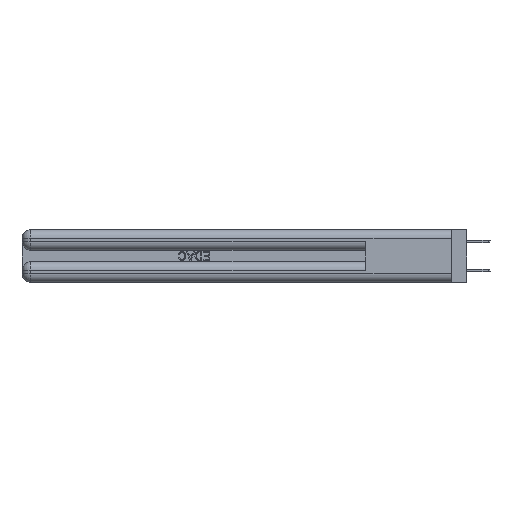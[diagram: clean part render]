
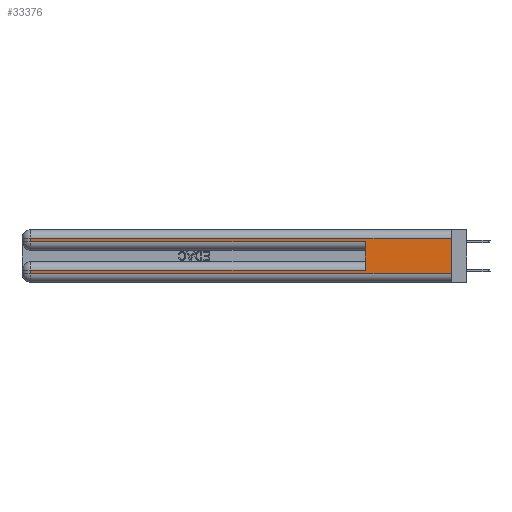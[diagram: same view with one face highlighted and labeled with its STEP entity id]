
A CAD part, left-side view. The second image highlights one B-rep face of the part: STEP entity #33376.
In plain terms, the highlighted planar face has unit normal (-1, 0, 0).
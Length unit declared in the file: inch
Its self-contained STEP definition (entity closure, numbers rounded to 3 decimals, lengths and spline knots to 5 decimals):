
#803 = LINE ( 'NONE', #3390, #34950 ) ;
#2134 = CARTESIAN_POINT ( 'NONE',  ( 0., 2.94, 0.085 ) ) ;
#2688 = VERTEX_POINT ( 'NONE', #10606 ) ;
#3357 = VECTOR ( 'NONE', #13392, 39.37008 ) ;
#3390 = CARTESIAN_POINT ( 'NONE',  ( 0., 0., 0.31 ) ) ;
#4240 = CARTESIAN_POINT ( 'NONE',  ( 0., 0., 0.37 ) ) ;
#5053 = CARTESIAN_POINT ( 'NONE',  ( 0., 2.94, 0.285 ) ) ;
#6180 = EDGE_CURVE ( 'NONE', #27935, #36361, #23320, .T. ) ;
#6785 = DIRECTION ( 'NONE',  ( 0., 1., 0. ) ) ;
#7603 = DIRECTION ( 'NONE',  ( 0., 0., -1. ) ) ;
#8574 = ORIENTED_EDGE ( 'NONE', *, *, #15622, .T. ) ;
#8674 = ORIENTED_EDGE ( 'NONE', *, *, #22740, .F. ) ;
#9617 = DIRECTION ( 'NONE',  ( 0., -1., 0. ) ) ;
#10099 = CARTESIAN_POINT ( 'NONE',  ( 0., 0.6, 0.145 ) ) ;
#10606 = CARTESIAN_POINT ( 'NONE',  ( 0., 0., 0.06 ) ) ;
#11550 = VERTEX_POINT ( 'NONE', #33632 ) ;
#13392 = DIRECTION ( 'NONE',  ( 0., 0., 1. ) ) ;
#14465 = CARTESIAN_POINT ( 'NONE',  ( 0., 2.94, 0.37 ) ) ;
#15622 = EDGE_CURVE ( 'NONE', #24489, #27935, #23528, .T. ) ;
#15987 = VERTEX_POINT ( 'NONE', #23388 ) ;
#16885 = CARTESIAN_POINT ( 'NONE',  ( 0., 0., 0.31 ) ) ;
#17407 = PLANE ( 'NONE',  #38671 ) ;
#17428 = DIRECTION ( 'NONE',  ( 0., 1., 0. ) ) ;
#18054 = EDGE_CURVE ( 'NONE', #36361, #2688, #40770, .T. ) ;
#18984 = ORIENTED_EDGE ( 'NONE', *, *, #21351, .T. ) ;
#19740 = LINE ( 'NONE', #29223, #36273 ) ;
#21266 = VECTOR ( 'NONE', #34198, 39.37008 ) ;
#21351 = EDGE_CURVE ( 'NONE', #11550, #28481, #19740, .T. ) ;
#22107 = FACE_OUTER_BOUND ( 'NONE', #23478, .T. ) ;
#22740 = EDGE_CURVE ( 'NONE', #38735, #2688, #38508, .T. ) ;
#23072 = VECTOR ( 'NONE', #37963, 39.37008 ) ;
#23320 = LINE ( 'NONE', #14465, #21266 ) ;
#23343 = CARTESIAN_POINT ( 'NONE',  ( 0., 0., 0.37 ) ) ;
#23388 = CARTESIAN_POINT ( 'NONE',  ( 0., 0.6, 0.285 ) ) ;
#23475 = DIRECTION ( 'NONE',  ( 0., 0., -1. ) ) ;
#23478 = EDGE_LOOP ( 'NONE', ( #8674, #36290, #18984, #28076, #25485, #8574, #33791, #26164 ) ) ;
#23528 = LINE ( 'NONE', #40569, #41222 ) ;
#24489 = VERTEX_POINT ( 'NONE', #25614 ) ;
#24587 = CARTESIAN_POINT ( 'NONE',  ( 0., 0., 0.06 ) ) ;
#25485 = ORIENTED_EDGE ( 'NONE', *, *, #28805, .F. ) ;
#25614 = CARTESIAN_POINT ( 'NONE',  ( 0., 0.6, 0.085 ) ) ;
#25879 = DIRECTION ( 'NONE',  ( 0., 0., -1. ) ) ;
#26164 = ORIENTED_EDGE ( 'NONE', *, *, #18054, .T. ) ;
#27282 = DIRECTION ( 'NONE',  ( 1., 0., 0. ) ) ;
#27935 = VERTEX_POINT ( 'NONE', #2134 ) ;
#28076 = ORIENTED_EDGE ( 'NONE', *, *, #31022, .T. ) ;
#28481 = VERTEX_POINT ( 'NONE', #5053 ) ;
#28654 = LINE ( 'NONE', #10099, #3357 ) ;
#28805 = EDGE_CURVE ( 'NONE', #24489, #15987, #28654, .T. ) ;
#29223 = CARTESIAN_POINT ( 'NONE',  ( 0., 2.94, 0.37 ) ) ;
#31022 = EDGE_CURVE ( 'NONE', #28481, #15987, #33168, .T. ) ;
#33168 = LINE ( 'NONE', #42577, #34218 ) ;
#33376 = ADVANCED_FACE ( 'NONE', ( #22107 ), #17407, .F. ) ;
#33632 = CARTESIAN_POINT ( 'NONE',  ( 0., 2.94, 0.31 ) ) ;
#33791 = ORIENTED_EDGE ( 'NONE', *, *, #6180, .T. ) ;
#34198 = DIRECTION ( 'NONE',  ( 0., 0., -1. ) ) ;
#34218 = VECTOR ( 'NONE', #9617, 39.37008 ) ;
#34659 = EDGE_CURVE ( 'NONE', #38735, #11550, #803, .T. ) ;
#34950 = VECTOR ( 'NONE', #6785, 39.37008 ) ;
#36273 = VECTOR ( 'NONE', #25879, 39.37008 ) ;
#36290 = ORIENTED_EDGE ( 'NONE', *, *, #34659, .T. ) ;
#36361 = VERTEX_POINT ( 'NONE', #40742 ) ;
#37449 = VECTOR ( 'NONE', #23475, 39.37008 ) ;
#37963 = DIRECTION ( 'NONE',  ( 0., -1., 0. ) ) ;
#38508 = LINE ( 'NONE', #23343, #37449 ) ;
#38671 = AXIS2_PLACEMENT_3D ( 'NONE', #4240, #27282, #7603 ) ;
#38735 = VERTEX_POINT ( 'NONE', #16885 ) ;
#40569 = CARTESIAN_POINT ( 'NONE',  ( 0., 0., 0.085 ) ) ;
#40742 = CARTESIAN_POINT ( 'NONE',  ( 0., 2.94, 0.06 ) ) ;
#40770 = LINE ( 'NONE', #24587, #23072 ) ;
#41222 = VECTOR ( 'NONE', #17428, 39.37008 ) ;
#42577 = CARTESIAN_POINT ( 'NONE',  ( 0., 0., 0.285 ) ) ;
